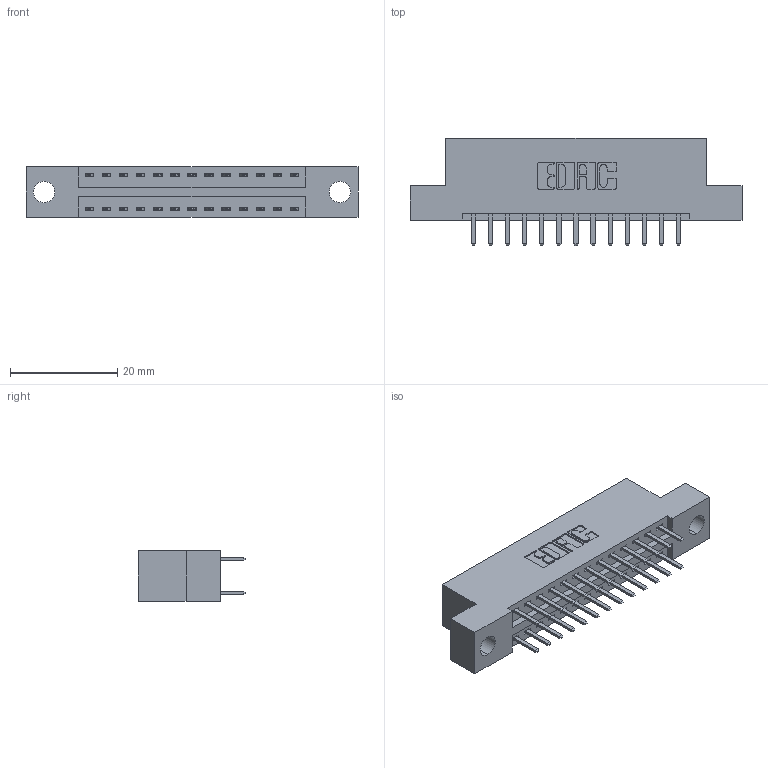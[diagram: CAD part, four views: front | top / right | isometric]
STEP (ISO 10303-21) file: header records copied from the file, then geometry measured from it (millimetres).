
FILE_DESCRIPTION (( 'STEP AP203' ), '1' );
FILE_NAME ('346-026-520-204.STEP', '2022-05-19T01:03:06', ( '' ), ( '' ), 'SwSTEP 2.0', 'SolidWorks 2020', '' );
FILE_SCHEMA (( 'CONFIG_CONTROL_DESIGN' ));
Length unit declared in the file: inch
Products named in the file (3): 345-292-001_345-293-120; 346-026-520-204; 346 Part_Flush Mounting Lugs - 0.156 Dia-TH
Assembly tree (27 placements, depth 2):
  346-026-520-204
    346 Part_Flush Mounting Lugs - 0.156 Dia-TH
    345-292-001_345-293-120  x26
Bounding box: 61.85 x 20.02 x 9.4 mm (x, y, z)
Volume: 5688.4 mm3; surface area: 7184.4 mm2
Topology: 27 solids, 27 shells, 1592 faces, 4603 edges, 2998 vertices
Faces by surface type: plane 1052, cylinder 540
Entity records: 12921 total; most frequent: CARTESIAN_POINT 2186, ORIENTED_EDGE 2106, DIRECTION 1965, EDGE_CURVE 1053, VECTOR 865, LINE 865, VERTEX_POINT 698, AXIS2_PLACEMENT_3D 550
